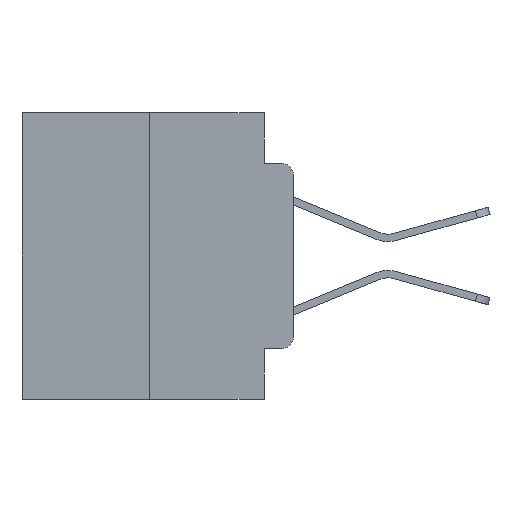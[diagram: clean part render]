
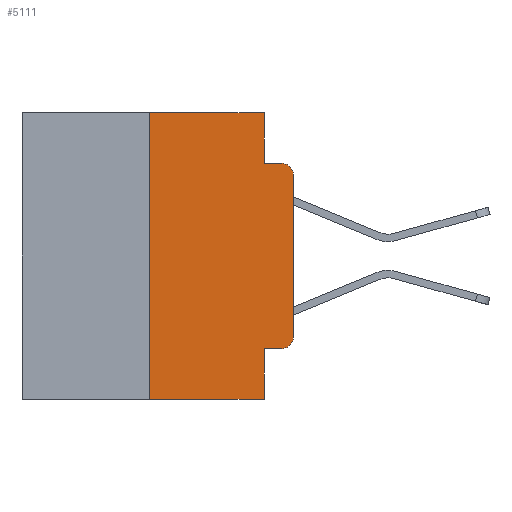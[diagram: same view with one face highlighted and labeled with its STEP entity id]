
A CAD part, left-side view. The second image highlights one B-rep face of the part: STEP entity #5111.
In plain terms, the highlighted planar face has unit normal (-1, 0, 0).
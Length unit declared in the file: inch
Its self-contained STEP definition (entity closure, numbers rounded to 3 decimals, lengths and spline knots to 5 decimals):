
#284 = LINE ( 'NONE', #20611, #17122 ) ;
#746 = VECTOR ( 'NONE', #24912, 39.37008 ) ;
#757 = EDGE_CURVE ( 'NONE', #11675, #16924, #9728, .T. ) ;
#899 = LINE ( 'NONE', #1871, #17719 ) ;
#1257 = CARTESIAN_POINT ( 'NONE',  ( 0., 0.473, 0. ) ) ;
#1871 = CARTESIAN_POINT ( 'NONE',  ( 0., 0.051, -0.0885 ) ) ;
#2293 = EDGE_CURVE ( 'NONE', #18258, #2414, #17054, .T. ) ;
#2414 = VERTEX_POINT ( 'NONE', #7633 ) ;
#2697 = EDGE_CURVE ( 'NONE', #19768, #27165, #899, .T. ) ;
#3064 = LINE ( 'NONE', #26336, #8946 ) ;
#3378 = ORIENTED_EDGE ( 'NONE', *, *, #20429, .T. ) ;
#3483 = CARTESIAN_POINT ( 'NONE',  ( 0., 0.02, -0.1085 ) ) ;
#3487 = ORIENTED_EDGE ( 'NONE', *, *, #2293, .F. ) ;
#3661 = ORIENTED_EDGE ( 'NONE', *, *, #16651, .F. ) ;
#4195 = DIRECTION ( 'NONE',  ( 0., -1., 0. ) ) ;
#4737 = CARTESIAN_POINT ( 'NONE',  ( 0., 0.25, -0.5 ) ) ;
#4998 = ORIENTED_EDGE ( 'NONE', *, *, #9183, .F. ) ;
#5077 = ORIENTED_EDGE ( 'NONE', *, *, #2697, .F. ) ;
#5111 = ADVANCED_FACE ( 'NONE', ( #23048 ), #23137, .F. ) ;
#5278 = ORIENTED_EDGE ( 'NONE', *, *, #757, .F. ) ;
#5624 = DIRECTION ( 'NONE',  ( -1., 0., 0. ) ) ;
#5713 = DIRECTION ( 'NONE',  ( 0., 0., -1. ) ) ;
#5984 = VERTEX_POINT ( 'NONE', #9898 ) ;
#6042 = VERTEX_POINT ( 'NONE', #27443 ) ;
#6915 = CARTESIAN_POINT ( 'NONE',  ( 0., 0.051, -0.4115 ) ) ;
#6949 = DIRECTION ( 'NONE',  ( 0., 0., -1. ) ) ;
#7545 = CARTESIAN_POINT ( 'NONE',  ( 0., 0.051, -0.0885 ) ) ;
#7564 = CIRCLE ( 'NONE', #22754, 0.02 ) ;
#7583 = CARTESIAN_POINT ( 'NONE',  ( 0., 0.473, 0. ) ) ;
#7633 = CARTESIAN_POINT ( 'NONE',  ( 0., 0.25, 0. ) ) ;
#7800 = EDGE_CURVE ( 'NONE', #18258, #16924, #284, .T. ) ;
#8111 = EDGE_LOOP ( 'NONE', ( #18208, #15292, #5077, #4998, #3661, #3487, #16613, #5278, #16342, #3378 ) ) ;
#8793 = DIRECTION ( 'NONE',  ( 0., 0., -1. ) ) ;
#8946 = VECTOR ( 'NONE', #11182, 39.37008 ) ;
#9063 = VECTOR ( 'NONE', #8793, 39.37008 ) ;
#9183 = EDGE_CURVE ( 'NONE', #12824, #19768, #23189, .T. ) ;
#9285 = AXIS2_PLACEMENT_3D ( 'NONE', #3483, #18704, #5713 ) ;
#9728 = LINE ( 'NONE', #23914, #9063 ) ;
#9898 = CARTESIAN_POINT ( 'NONE',  ( 0., 0.02, -0.4115 ) ) ;
#10166 = DIRECTION ( 'NONE',  ( 1., 0., 0. ) ) ;
#11182 = DIRECTION ( 'NONE',  ( 0., 0., 1. ) ) ;
#11295 = VECTOR ( 'NONE', #18069, 39.37008 ) ;
#11675 = VERTEX_POINT ( 'NONE', #6915 ) ;
#12824 = VERTEX_POINT ( 'NONE', #25007 ) ;
#13344 = CARTESIAN_POINT ( 'NONE',  ( 0., 0.02, -0.0885 ) ) ;
#14746 = DIRECTION ( 'NONE',  ( 0., -1., 0. ) ) ;
#15159 = CARTESIAN_POINT ( 'NONE',  ( 0., 0.051, -0.5 ) ) ;
#15292 = ORIENTED_EDGE ( 'NONE', *, *, #17872, .T. ) ;
#15895 = CARTESIAN_POINT ( 'NONE',  ( 0., 0.25, 0. ) ) ;
#16342 = ORIENTED_EDGE ( 'NONE', *, *, #27608, .T. ) ;
#16613 = ORIENTED_EDGE ( 'NONE', *, *, #7800, .T. ) ;
#16651 = EDGE_CURVE ( 'NONE', #2414, #12824, #23333, .T. ) ;
#16924 = VERTEX_POINT ( 'NONE', #15159 ) ;
#17054 = LINE ( 'NONE', #15895, #11295 ) ;
#17122 = VECTOR ( 'NONE', #22759, 39.37008 ) ;
#17427 = VECTOR ( 'NONE', #6949, 39.37008 ) ;
#17719 = VECTOR ( 'NONE', #4195, 39.37008 ) ;
#17754 = CARTESIAN_POINT ( 'NONE',  ( 0., 0.051, 0. ) ) ;
#17872 = EDGE_CURVE ( 'NONE', #18691, #27165, #19567, .T. ) ;
#18069 = DIRECTION ( 'NONE',  ( 0., 0., 1. ) ) ;
#18208 = ORIENTED_EDGE ( 'NONE', *, *, #20811, .T. ) ;
#18258 = VERTEX_POINT ( 'NONE', #4737 ) ;
#18617 = CARTESIAN_POINT ( 'NONE',  ( 0., 0.02, -0.3915 ) ) ;
#18691 = VERTEX_POINT ( 'NONE', #21709 ) ;
#18704 = DIRECTION ( 'NONE',  ( -1., 0., 0. ) ) ;
#19117 = CARTESIAN_POINT ( 'NONE',  ( 0., 0.051, -0.4115 ) ) ;
#19567 = CIRCLE ( 'NONE', #9285, 0.02 ) ;
#19768 = VERTEX_POINT ( 'NONE', #7545 ) ;
#20429 = EDGE_CURVE ( 'NONE', #5984, #6042, #7564, .T. ) ;
#20611 = CARTESIAN_POINT ( 'NONE',  ( 0., 0.473, -0.5 ) ) ;
#20811 = EDGE_CURVE ( 'NONE', #6042, #18691, #3064, .T. ) ;
#20818 = DIRECTION ( 'NONE',  ( 0., 0., -1. ) ) ;
#20885 = AXIS2_PLACEMENT_3D ( 'NONE', #1257, #10166, #25305 ) ;
#21709 = CARTESIAN_POINT ( 'NONE',  ( 0., 0., -0.1085 ) ) ;
#22754 = AXIS2_PLACEMENT_3D ( 'NONE', #18617, #5624, #20818 ) ;
#22759 = DIRECTION ( 'NONE',  ( 0., -1., 0. ) ) ;
#23048 = FACE_OUTER_BOUND ( 'NONE', #8111, .T. ) ;
#23137 = PLANE ( 'NONE',  #20885 ) ;
#23189 = LINE ( 'NONE', #17754, #17427 ) ;
#23333 = LINE ( 'NONE', #7583, #746 ) ;
#23914 = CARTESIAN_POINT ( 'NONE',  ( 0., 0.051, 0. ) ) ;
#24912 = DIRECTION ( 'NONE',  ( 0., -1., 0. ) ) ;
#25007 = CARTESIAN_POINT ( 'NONE',  ( 0., 0.051, 0. ) ) ;
#25305 = DIRECTION ( 'NONE',  ( 0., 0., -1. ) ) ;
#26336 = CARTESIAN_POINT ( 'NONE',  ( 0., 0., 0. ) ) ;
#27161 = VECTOR ( 'NONE', #14746, 39.37008 ) ;
#27165 = VERTEX_POINT ( 'NONE', #13344 ) ;
#27443 = CARTESIAN_POINT ( 'NONE',  ( 0., 0., -0.3915 ) ) ;
#27608 = EDGE_CURVE ( 'NONE', #11675, #5984, #27824, .T. ) ;
#27824 = LINE ( 'NONE', #19117, #27161 ) ;
